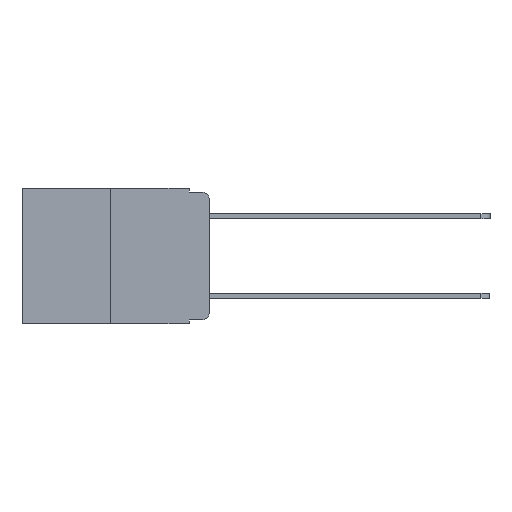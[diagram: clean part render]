
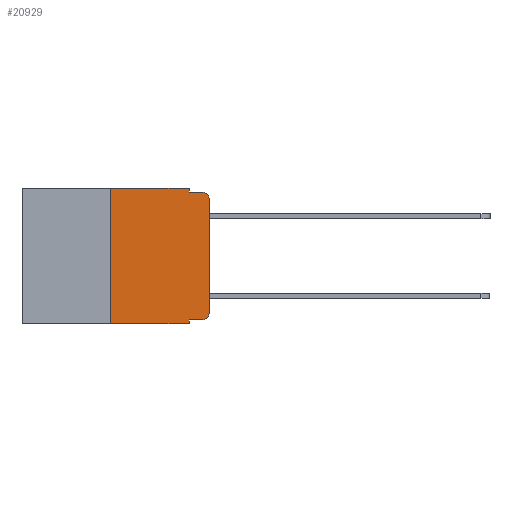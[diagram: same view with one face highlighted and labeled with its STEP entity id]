
A CAD part, left-side view. The second image highlights one B-rep face of the part: STEP entity #20929.
In plain terms, the highlighted planar face has unit normal (-1, 0, 0).
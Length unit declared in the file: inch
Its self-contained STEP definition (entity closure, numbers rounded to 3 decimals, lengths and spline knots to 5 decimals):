
#465 = AXIS2_PLACEMENT_3D ( 'NONE', #19904, #9054, #21686 ) ;
#579 = VECTOR ( 'NONE', #16264, 39.37008 ) ;
#597 = VECTOR ( 'NONE', #11839, 39.37008 ) ;
#908 = VERTEX_POINT ( 'NONE', #6316 ) ;
#1233 = EDGE_CURVE ( 'NONE', #13389, #908, #3096, .T. ) ;
#1542 = DIRECTION ( 'NONE',  ( 0., -1., 0. ) ) ;
#2001 = CARTESIAN_POINT ( 'NONE',  ( 0., 0.051, -0.01 ) ) ;
#2767 = CARTESIAN_POINT ( 'NONE',  ( 0., 0.02, -0.03 ) ) ;
#2790 = CARTESIAN_POINT ( 'NONE',  ( 0., 0., -0.03 ) ) ;
#2819 = EDGE_CURVE ( 'NONE', #16278, #12165, #17799, .T. ) ;
#3081 = ORIENTED_EDGE ( 'NONE', *, *, #9662, .F. ) ;
#3096 = CIRCLE ( 'NONE', #465, 0.02 ) ;
#3252 = VERTEX_POINT ( 'NONE', #2001 ) ;
#3605 = ORIENTED_EDGE ( 'NONE', *, *, #23390, .T. ) ;
#3648 = LINE ( 'NONE', #22364, #8535 ) ;
#3817 = ORIENTED_EDGE ( 'NONE', *, *, #14581, .T. ) ;
#4643 = DIRECTION ( 'NONE',  ( 0., 0., -1. ) ) ;
#4671 = EDGE_CURVE ( 'NONE', #6813, #3252, #6959, .T. ) ;
#4779 = AXIS2_PLACEMENT_3D ( 'NONE', #20299, #22070, #11266 ) ;
#5043 = ORIENTED_EDGE ( 'NONE', *, *, #2819, .F. ) ;
#5213 = CARTESIAN_POINT ( 'NONE',  ( 0., 0.02, -0.01 ) ) ;
#5533 = LINE ( 'NONE', #21604, #579 ) ;
#5614 = CARTESIAN_POINT ( 'NONE',  ( 0., 0.25, -0.343 ) ) ;
#5624 = LINE ( 'NONE', #19682, #18953 ) ;
#5885 = EDGE_LOOP ( 'NONE', ( #3817, #20538, #3081, #14035, #8172, #5043, #21907, #9306, #3605, #12987 ) ) ;
#6316 = CARTESIAN_POINT ( 'NONE',  ( 0., 0., -0.313 ) ) ;
#6377 = VECTOR ( 'NONE', #22963, 39.37008 ) ;
#6813 = VERTEX_POINT ( 'NONE', #18305 ) ;
#6959 = LINE ( 'NONE', #8645, #6377 ) ;
#7575 = CARTESIAN_POINT ( 'NONE',  ( 0., 0.051, 0. ) ) ;
#7826 = DIRECTION ( 'NONE',  ( 0., 0., 1. ) ) ;
#8117 = EDGE_CURVE ( 'NONE', #12379, #17382, #14712, .T. ) ;
#8172 = ORIENTED_EDGE ( 'NONE', *, *, #22285, .F. ) ;
#8535 = VECTOR ( 'NONE', #15211, 39.37008 ) ;
#8645 = CARTESIAN_POINT ( 'NONE',  ( 0., 0.051, 0. ) ) ;
#8761 = CARTESIAN_POINT ( 'NONE',  ( 0., 0.051, -0.333 ) ) ;
#9054 = DIRECTION ( 'NONE',  ( -1., 0., 0. ) ) ;
#9187 = CARTESIAN_POINT ( 'NONE',  ( 0., 0.25, 0. ) ) ;
#9306 = ORIENTED_EDGE ( 'NONE', *, *, #8117, .F. ) ;
#9372 = DIRECTION ( 'NONE',  ( 0., 0., -1. ) ) ;
#9662 = EDGE_CURVE ( 'NONE', #3252, #13572, #5624, .T. ) ;
#10200 = LINE ( 'NONE', #20402, #19275 ) ;
#11266 = DIRECTION ( 'NONE',  ( 0., 0., -1. ) ) ;
#11359 = CIRCLE ( 'NONE', #13148, 0.02 ) ;
#11369 = DIRECTION ( 'NONE',  ( 0., -1., 0. ) ) ;
#11839 = DIRECTION ( 'NONE',  ( 0., -1., 0. ) ) ;
#12165 = VERTEX_POINT ( 'NONE', #9187 ) ;
#12379 = VERTEX_POINT ( 'NONE', #8761 ) ;
#12987 = ORIENTED_EDGE ( 'NONE', *, *, #1233, .T. ) ;
#13148 = AXIS2_PLACEMENT_3D ( 'NONE', #2767, #15484, #4643 ) ;
#13389 = VERTEX_POINT ( 'NONE', #17351 ) ;
#13572 = VERTEX_POINT ( 'NONE', #5213 ) ;
#14003 = EDGE_CURVE ( 'NONE', #16609, #13572, #11359, .T. ) ;
#14035 = ORIENTED_EDGE ( 'NONE', *, *, #4671, .F. ) ;
#14581 = EDGE_CURVE ( 'NONE', #908, #16609, #3648, .T. ) ;
#14712 = LINE ( 'NONE', #7575, #15291 ) ;
#15171 = LINE ( 'NONE', #20878, #597 ) ;
#15211 = DIRECTION ( 'NONE',  ( 0., 0., 1. ) ) ;
#15291 = VECTOR ( 'NONE', #9372, 39.37008 ) ;
#15484 = DIRECTION ( 'NONE',  ( -1., 0., 0. ) ) ;
#16264 = DIRECTION ( 'NONE',  ( 0., -1., 0. ) ) ;
#16278 = VERTEX_POINT ( 'NONE', #5614 ) ;
#16609 = VERTEX_POINT ( 'NONE', #2790 ) ;
#16973 = FACE_OUTER_BOUND ( 'NONE', #5885, .T. ) ;
#17351 = CARTESIAN_POINT ( 'NONE',  ( 0., 0.02, -0.333 ) ) ;
#17382 = VERTEX_POINT ( 'NONE', #22273 ) ;
#17799 = LINE ( 'NONE', #18668, #21992 ) ;
#18305 = CARTESIAN_POINT ( 'NONE',  ( 0., 0.051, 0. ) ) ;
#18493 = PLANE ( 'NONE',  #4779 ) ;
#18668 = CARTESIAN_POINT ( 'NONE',  ( 0., 0.25, 0. ) ) ;
#18953 = VECTOR ( 'NONE', #1542, 39.37008 ) ;
#19275 = VECTOR ( 'NONE', #11369, 39.37008 ) ;
#19682 = CARTESIAN_POINT ( 'NONE',  ( 0., 0.051, -0.01 ) ) ;
#19904 = CARTESIAN_POINT ( 'NONE',  ( 0., 0.02, -0.313 ) ) ;
#20299 = CARTESIAN_POINT ( 'NONE',  ( 0., 0.473, 0. ) ) ;
#20374 = EDGE_CURVE ( 'NONE', #16278, #17382, #10200, .T. ) ;
#20402 = CARTESIAN_POINT ( 'NONE',  ( 0., 0.473, -0.343 ) ) ;
#20538 = ORIENTED_EDGE ( 'NONE', *, *, #14003, .T. ) ;
#20878 = CARTESIAN_POINT ( 'NONE',  ( 0., 0.473, 0. ) ) ;
#20929 = ADVANCED_FACE ( 'NONE', ( #16973 ), #18493, .F. ) ;
#21604 = CARTESIAN_POINT ( 'NONE',  ( 0., 0.051, -0.333 ) ) ;
#21686 = DIRECTION ( 'NONE',  ( 0., 0., -1. ) ) ;
#21907 = ORIENTED_EDGE ( 'NONE', *, *, #20374, .T. ) ;
#21992 = VECTOR ( 'NONE', #7826, 39.37008 ) ;
#22070 = DIRECTION ( 'NONE',  ( 1., 0., 0. ) ) ;
#22273 = CARTESIAN_POINT ( 'NONE',  ( 0., 0.051, -0.343 ) ) ;
#22285 = EDGE_CURVE ( 'NONE', #12165, #6813, #15171, .T. ) ;
#22364 = CARTESIAN_POINT ( 'NONE',  ( 0., 0., 0. ) ) ;
#22963 = DIRECTION ( 'NONE',  ( 0., 0., -1. ) ) ;
#23390 = EDGE_CURVE ( 'NONE', #12379, #13389, #5533, .T. ) ;
